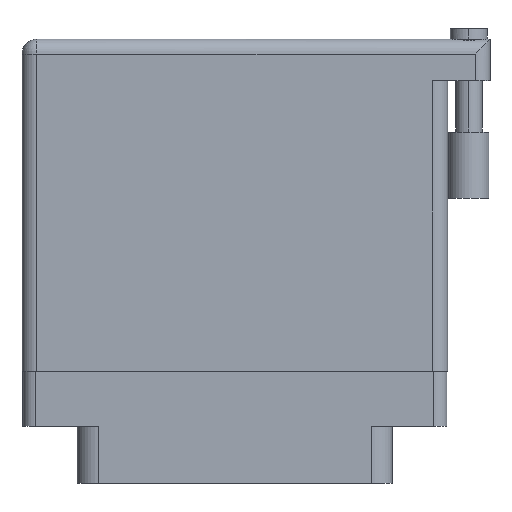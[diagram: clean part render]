
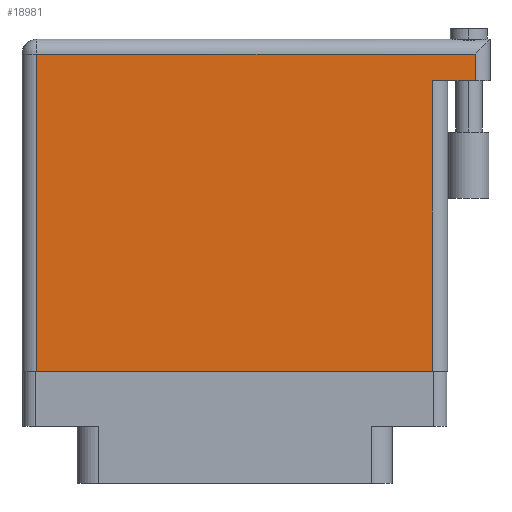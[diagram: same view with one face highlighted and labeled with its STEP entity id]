
A CAD part, front view. The second image highlights one B-rep face of the part: STEP entity #18981.
In plain terms, the highlighted face is planar.
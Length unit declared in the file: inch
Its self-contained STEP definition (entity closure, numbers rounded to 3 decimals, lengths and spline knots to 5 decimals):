
#465 = LINE ( 'NONE', #6443, #28279 ) ;
#1420 = VERTEX_POINT ( 'NONE', #32509 ) ;
#1895 = VECTOR ( 'NONE', #11499, 39.37008 ) ;
#2086 = VERTEX_POINT ( 'NONE', #31302 ) ;
#2931 = CARTESIAN_POINT ( 'NONE',  ( 1.938, 0., 0. ) ) ;
#5244 = ORIENTED_EDGE ( 'NONE', *, *, #24143, .T. ) ;
#5960 = CARTESIAN_POINT ( 'NONE',  ( 0.07, 1.496, 0. ) ) ;
#6395 = LINE ( 'NONE', #25931, #19070 ) ;
#6443 = CARTESIAN_POINT ( 'NONE',  ( 2.208, 1.369, 0. ) ) ;
#6994 = CARTESIAN_POINT ( 'NONE',  ( 0.07, 0., 0. ) ) ;
#7477 = EDGE_CURVE ( 'NONE', #1420, #2086, #27570, .T. ) ;
#7801 = ORIENTED_EDGE ( 'NONE', *, *, #16237, .F. ) ;
#8546 = DIRECTION ( 'NONE',  ( 0., -1., 0. ) ) ;
#9147 = VERTEX_POINT ( 'NONE', #26222 ) ;
#11499 = DIRECTION ( 'NONE',  ( -1., 0., 0. ) ) ;
#11656 = VERTEX_POINT ( 'NONE', #5960 ) ;
#12115 = CARTESIAN_POINT ( 'NONE',  ( 1.938, 1.369, 0. ) ) ;
#13226 = EDGE_LOOP ( 'NONE', ( #27081, #34421, #7801, #32364, #5244, #14297 ) ) ;
#13756 = PLANE ( 'NONE',  #22178 ) ;
#14297 = ORIENTED_EDGE ( 'NONE', *, *, #26747, .T. ) ;
#14480 = VECTOR ( 'NONE', #8546, 39.37008 ) ;
#15103 = DIRECTION ( 'NONE',  ( 0., 1., 0. ) ) ;
#16237 = EDGE_CURVE ( 'NONE', #1420, #9147, #465, .T. ) ;
#17283 = DIRECTION ( 'NONE',  ( -1., 0., 0. ) ) ;
#17924 = DIRECTION ( 'NONE',  ( 0., 1., 0. ) ) ;
#18675 = LINE ( 'NONE', #12115, #32120 ) ;
#18981 = ADVANCED_FACE ( 'NONE', ( #25558 ), #13756, .F. ) ;
#19070 = VECTOR ( 'NONE', #31438, 39.37008 ) ;
#19162 = VECTOR ( 'NONE', #15103, 39.37008 ) ;
#19316 = DIRECTION ( 'NONE',  ( -1., 0., 0. ) ) ;
#20874 = VERTEX_POINT ( 'NONE', #6994 ) ;
#21705 = CARTESIAN_POINT ( 'NONE',  ( 0., 1.566, 0. ) ) ;
#22040 = DIRECTION ( 'NONE',  ( 0., 0., -1. ) ) ;
#22178 = AXIS2_PLACEMENT_3D ( 'NONE', #21705, #22040, #19316 ) ;
#24143 = EDGE_CURVE ( 'NONE', #2086, #11656, #33893, .T. ) ;
#25558 = FACE_OUTER_BOUND ( 'NONE', #13226, .T. ) ;
#25931 = CARTESIAN_POINT ( 'NONE',  ( 0., 0., 0. ) ) ;
#26222 = CARTESIAN_POINT ( 'NONE',  ( 1.938, 1.369, 0. ) ) ;
#26747 = EDGE_CURVE ( 'NONE', #11656, #20874, #34266, .T. ) ;
#26968 = CARTESIAN_POINT ( 'NONE',  ( 0.07, 0., 0. ) ) ;
#27081 = ORIENTED_EDGE ( 'NONE', *, *, #27573, .T. ) ;
#27470 = EDGE_CURVE ( 'NONE', #31683, #9147, #18675, .T. ) ;
#27570 = LINE ( 'NONE', #28422, #19162 ) ;
#27573 = EDGE_CURVE ( 'NONE', #20874, #31683, #6395, .T. ) ;
#28279 = VECTOR ( 'NONE', #17283, 39.37008 ) ;
#28422 = CARTESIAN_POINT ( 'NONE',  ( 2.138, 1.566, 0. ) ) ;
#30011 = CARTESIAN_POINT ( 'NONE',  ( 0., 1.496, 0. ) ) ;
#31302 = CARTESIAN_POINT ( 'NONE',  ( 2.138, 1.496, 0. ) ) ;
#31438 = DIRECTION ( 'NONE',  ( 1., 0., 0. ) ) ;
#31683 = VERTEX_POINT ( 'NONE', #2931 ) ;
#32120 = VECTOR ( 'NONE', #17924, 39.37008 ) ;
#32364 = ORIENTED_EDGE ( 'NONE', *, *, #7477, .T. ) ;
#32509 = CARTESIAN_POINT ( 'NONE',  ( 2.138, 1.369, 0. ) ) ;
#33893 = LINE ( 'NONE', #30011, #1895 ) ;
#34266 = LINE ( 'NONE', #26968, #14480 ) ;
#34421 = ORIENTED_EDGE ( 'NONE', *, *, #27470, .T. ) ;
